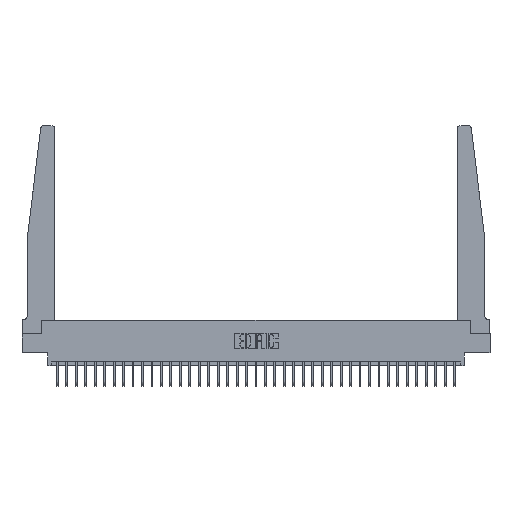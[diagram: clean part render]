
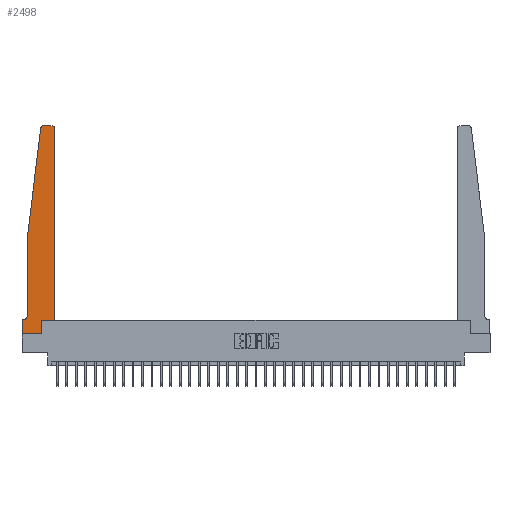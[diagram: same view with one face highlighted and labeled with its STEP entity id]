
A CAD part, top view. The second image highlights one B-rep face of the part: STEP entity #2498.
In plain terms, the highlighted planar face has unit normal (0, 0, 1).
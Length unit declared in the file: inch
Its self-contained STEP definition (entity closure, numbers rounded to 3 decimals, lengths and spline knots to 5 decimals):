
#108 = VECTOR ( 'NONE', #5866, 39.37008 ) ;
#203 = CARTESIAN_POINT ( 'NONE',  ( 0., 0.1875, 0.37 ) ) ;
#1340 = CARTESIAN_POINT ( 'NONE',  ( 0.27653, 2.75, 0.37 ) ) ;
#1416 = VERTEX_POINT ( 'NONE', #7482 ) ;
#1653 = AXIS2_PLACEMENT_3D ( 'NONE', #203, #2669, #19764 ) ;
#1665 = EDGE_CURVE ( 'NONE', #16850, #22720, #6676, .T. ) ;
#1712 = VERTEX_POINT ( 'NONE', #25669 ) ;
#1844 = VECTOR ( 'NONE', #4938, 39.37008 ) ;
#1982 = VERTEX_POINT ( 'NONE', #2382 ) ;
#2382 = CARTESIAN_POINT ( 'NONE',  ( 0.425, 2.72, 0.37 ) ) ;
#2498 = ADVANCED_FACE ( 'NONE', ( #11191 ), #26974, .T. ) ;
#2651 = EDGE_CURVE ( 'NONE', #1982, #5490, #31326, .T. ) ;
#2669 = DIRECTION ( 'NONE',  ( 0., 0., 1. ) ) ;
#3405 = ORIENTED_EDGE ( 'NONE', *, *, #18143, .T. ) ;
#4220 = ORIENTED_EDGE ( 'NONE', *, *, #2651, .T. ) ;
#4771 = CARTESIAN_POINT ( 'NONE',  ( 0.395, 2.75, 0.37 ) ) ;
#4938 = DIRECTION ( 'NONE',  ( 0., -1., 0. ) ) ;
#5434 = LINE ( 'NONE', #15912, #16857 ) ;
#5490 = VERTEX_POINT ( 'NONE', #4771 ) ;
#5866 = DIRECTION ( 'NONE',  ( 0., -1., 0. ) ) ;
#6095 = VECTOR ( 'NONE', #17530, 39.37008 ) ;
#6272 = EDGE_CURVE ( 'NONE', #12236, #16850, #14008, .T. ) ;
#6551 = VERTEX_POINT ( 'NONE', #1340 ) ;
#6617 = LINE ( 'NONE', #20243, #24519 ) ;
#6676 = LINE ( 'NONE', #22927, #108 ) ;
#7395 = CARTESIAN_POINT ( 'NONE',  ( 0., 0., 0.37 ) ) ;
#7472 = CARTESIAN_POINT ( 'NONE',  ( 0.2605, 0., 0.37 ) ) ;
#7482 = CARTESIAN_POINT ( 'NONE',  ( 0., 0.1875, 0.37 ) ) ;
#7501 = CARTESIAN_POINT ( 'NONE',  ( 0.065, 0.2375, 0.37 ) ) ;
#7599 = CARTESIAN_POINT ( 'NONE',  ( 0.065, 1.25, 0.37 ) ) ;
#7647 = VECTOR ( 'NONE', #15596, 39.37008 ) ;
#8329 = VECTOR ( 'NONE', #22219, 39.37008 ) ;
#8388 = LINE ( 'NONE', #7395, #1844 ) ;
#8805 = ORIENTED_EDGE ( 'NONE', *, *, #12728, .T. ) ;
#8830 = EDGE_CURVE ( 'NONE', #5490, #6551, #6617, .T. ) ;
#9575 = ORIENTED_EDGE ( 'NONE', *, *, #15720, .T. ) ;
#9972 = DIRECTION ( 'NONE',  ( 0., 0., -1. ) ) ;
#10598 = CARTESIAN_POINT ( 'NONE',  ( 0.395, 2.72, 0.37 ) ) ;
#10694 = ORIENTED_EDGE ( 'NONE', *, *, #26566, .T. ) ;
#11191 = FACE_OUTER_BOUND ( 'NONE', #24688, .T. ) ;
#11504 = AXIS2_PLACEMENT_3D ( 'NONE', #10598, #27583, #13027 ) ;
#12003 = CARTESIAN_POINT ( 'NONE',  ( 0.065, 0.1875, 0.37 ) ) ;
#12236 = VERTEX_POINT ( 'NONE', #21798 ) ;
#12728 = EDGE_CURVE ( 'NONE', #25896, #27228, #15877, .T. ) ;
#12850 = VECTOR ( 'NONE', #29001, 39.37008 ) ;
#12865 = DIRECTION ( 'NONE',  ( -1., 0., 0. ) ) ;
#12966 = ORIENTED_EDGE ( 'NONE', *, *, #15297, .T. ) ;
#13027 = DIRECTION ( 'NONE',  ( 1., 0., 0. ) ) ;
#13244 = DIRECTION ( 'NONE',  ( 0., 0., 1. ) ) ;
#14008 = LINE ( 'NONE', #7599, #8329 ) ;
#14091 = ORIENTED_EDGE ( 'NONE', *, *, #8830, .T. ) ;
#15076 = CARTESIAN_POINT ( 'NONE',  ( 0.425, 0.18, 0.37 ) ) ;
#15297 = EDGE_CURVE ( 'NONE', #27228, #1712, #20610, .T. ) ;
#15596 = DIRECTION ( 'NONE',  ( 0., 1., 0. ) ) ;
#15622 = ORIENTED_EDGE ( 'NONE', *, *, #6272, .T. ) ;
#15720 = EDGE_CURVE ( 'NONE', #1416, #25896, #8388, .T. ) ;
#15877 = LINE ( 'NONE', #21441, #28041 ) ;
#15912 = CARTESIAN_POINT ( 'NONE',  ( 0.425, 0.18, 0.37 ) ) ;
#16176 = VERTEX_POINT ( 'NONE', #16294 ) ;
#16294 = CARTESIAN_POINT ( 'NONE',  ( 0.015, 0.1875, 0.37 ) ) ;
#16392 = ORIENTED_EDGE ( 'NONE', *, *, #16937, .T. ) ;
#16850 = VERTEX_POINT ( 'NONE', #28370 ) ;
#16857 = VECTOR ( 'NONE', #30557, 39.37008 ) ;
#16937 = EDGE_CURVE ( 'NONE', #16176, #1416, #31448, .T. ) ;
#17530 = DIRECTION ( 'NONE',  ( 1., 0., 0. ) ) ;
#17923 = ORIENTED_EDGE ( 'NONE', *, *, #30938, .T. ) ;
#18143 = EDGE_CURVE ( 'NONE', #6551, #12236, #26549, .T. ) ;
#18775 = VERTEX_POINT ( 'NONE', #23284 ) ;
#19764 = DIRECTION ( 'NONE',  ( 1., 0., 0. ) ) ;
#19895 = CARTESIAN_POINT ( 'NONE',  ( 0., 0., 0.37 ) ) ;
#20243 = CARTESIAN_POINT ( 'NONE',  ( 0.25, 2.75, 0.37 ) ) ;
#20610 = LINE ( 'NONE', #25299, #7647 ) ;
#21441 = CARTESIAN_POINT ( 'NONE',  ( 0., 0., 0.37 ) ) ;
#21549 = DIRECTION ( 'NONE',  ( 1., 0., 0. ) ) ;
#21798 = CARTESIAN_POINT ( 'NONE',  ( 0.24675, 2.72367, 0.37 ) ) ;
#22219 = DIRECTION ( 'NONE',  ( -0.122, -0.992, 0. ) ) ;
#22457 = EDGE_CURVE ( 'NONE', #18775, #1982, #5434, .T. ) ;
#22720 = VERTEX_POINT ( 'NONE', #7501 ) ;
#22927 = CARTESIAN_POINT ( 'NONE',  ( 0.065, 1.25, 0.37 ) ) ;
#23284 = CARTESIAN_POINT ( 'NONE',  ( 0.425, 0.18, 0.37 ) ) ;
#24519 = VECTOR ( 'NONE', #12865, 39.37008 ) ;
#24557 = CARTESIAN_POINT ( 'NONE',  ( 0.015, 0.2375, 0.37 ) ) ;
#24688 = EDGE_LOOP ( 'NONE', ( #14091, #3405, #15622, #30048, #10694, #16392, #9575, #8805, #12966, #17923, #27419, #4220 ) ) ;
#25299 = CARTESIAN_POINT ( 'NONE',  ( 0.2605, 0.18, 0.37 ) ) ;
#25382 = CIRCLE ( 'NONE', #26593, 0.05 ) ;
#25444 = AXIS2_PLACEMENT_3D ( 'NONE', #27823, #13244, #30237 ) ;
#25521 = LINE ( 'NONE', #15076, #6095 ) ;
#25669 = CARTESIAN_POINT ( 'NONE',  ( 0.2605, 0.18, 0.37 ) ) ;
#25896 = VERTEX_POINT ( 'NONE', #19895 ) ;
#26549 = CIRCLE ( 'NONE', #25444, 0.03 ) ;
#26566 = EDGE_CURVE ( 'NONE', #22720, #16176, #25382, .T. ) ;
#26593 = AXIS2_PLACEMENT_3D ( 'NONE', #24557, #9972, #26960 ) ;
#26960 = DIRECTION ( 'NONE',  ( -1., 0., 0. ) ) ;
#26974 = PLANE ( 'NONE',  #1653 ) ;
#27228 = VERTEX_POINT ( 'NONE', #7472 ) ;
#27419 = ORIENTED_EDGE ( 'NONE', *, *, #22457, .T. ) ;
#27583 = DIRECTION ( 'NONE',  ( 0., 0., 1. ) ) ;
#27823 = CARTESIAN_POINT ( 'NONE',  ( 0.27653, 2.72, 0.37 ) ) ;
#28041 = VECTOR ( 'NONE', #21549, 39.37008 ) ;
#28370 = CARTESIAN_POINT ( 'NONE',  ( 0.065, 1.25, 0.37 ) ) ;
#29001 = DIRECTION ( 'NONE',  ( -1., 0., 0. ) ) ;
#30048 = ORIENTED_EDGE ( 'NONE', *, *, #1665, .T. ) ;
#30237 = DIRECTION ( 'NONE',  ( 1., 0., 0. ) ) ;
#30557 = DIRECTION ( 'NONE',  ( 0., 1., 0. ) ) ;
#30938 = EDGE_CURVE ( 'NONE', #1712, #18775, #25521, .T. ) ;
#31326 = CIRCLE ( 'NONE', #11504, 0.03 ) ;
#31448 = LINE ( 'NONE', #12003, #12850 ) ;
